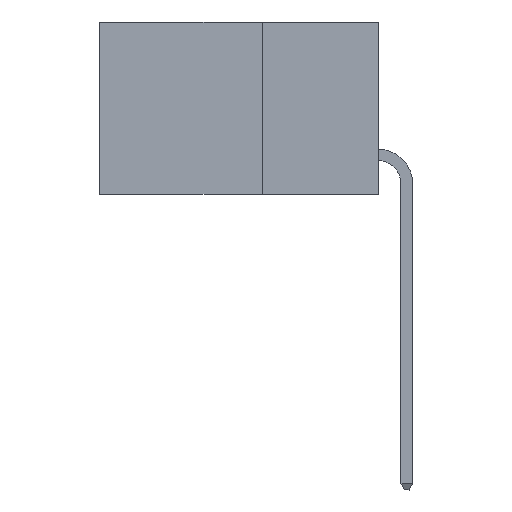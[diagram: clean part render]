
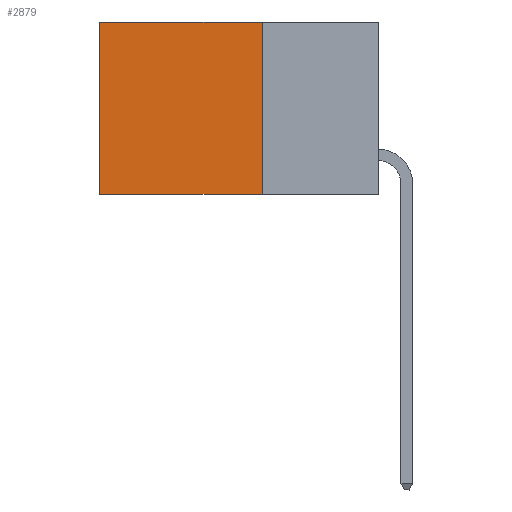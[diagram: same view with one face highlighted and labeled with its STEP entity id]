
A CAD part, left-side view. The second image highlights one B-rep face of the part: STEP entity #2879.
In plain terms, the highlighted planar face has unit normal (-1, 0, 0).
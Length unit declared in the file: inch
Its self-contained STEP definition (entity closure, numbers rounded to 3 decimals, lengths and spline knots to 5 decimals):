
#283 = ORIENTED_EDGE ( 'NONE', *, *, #8008, .T. ) ;
#364 = LINE ( 'NONE', #12319, #1823 ) ;
#633 = FACE_OUTER_BOUND ( 'NONE', #9803, .T. ) ;
#1013 = DIRECTION ( 'NONE',  ( 0., 1., 0. ) ) ;
#1372 = VERTEX_POINT ( 'NONE', #11351 ) ;
#1469 = VERTEX_POINT ( 'NONE', #7396 ) ;
#1823 = VECTOR ( 'NONE', #4928, 39.37008 ) ;
#2589 = DIRECTION ( 'NONE',  ( 0., 0., -1. ) ) ;
#2618 = ORIENTED_EDGE ( 'NONE', *, *, #8713, .F. ) ;
#2879 = ADVANCED_FACE ( 'NONE', ( #633 ), #7696, .F. ) ;
#3606 = VECTOR ( 'NONE', #6591, 39.37008 ) ;
#3637 = LINE ( 'NONE', #9438, #8852 ) ;
#4437 = VERTEX_POINT ( 'NONE', #12358 ) ;
#4906 = LINE ( 'NONE', #5611, #3606 ) ;
#4928 = DIRECTION ( 'NONE',  ( 0., 0., -1. ) ) ;
#5316 = DIRECTION ( 'NONE',  ( 0., 0., -1. ) ) ;
#5583 = DIRECTION ( 'NONE',  ( 1., 0., 0. ) ) ;
#5611 = CARTESIAN_POINT ( 'NONE',  ( 0.298, 0.25, 0. ) ) ;
#6186 = LINE ( 'NONE', #11544, #11407 ) ;
#6591 = DIRECTION ( 'NONE',  ( 0., 1., 0. ) ) ;
#7368 = EDGE_CURVE ( 'NONE', #4437, #1372, #4906, .T. ) ;
#7396 = CARTESIAN_POINT ( 'NONE',  ( 0.298, 0.6, -0.37 ) ) ;
#7447 = CARTESIAN_POINT ( 'NONE',  ( 0.298, 0.25, -0.37 ) ) ;
#7696 = PLANE ( 'NONE',  #12061 ) ;
#8008 = EDGE_CURVE ( 'NONE', #1372, #1469, #6186, .T. ) ;
#8713 = EDGE_CURVE ( 'NONE', #4437, #10358, #364, .T. ) ;
#8852 = VECTOR ( 'NONE', #1013, 39.37008 ) ;
#9438 = CARTESIAN_POINT ( 'NONE',  ( 0.298, 0.25, -0.37 ) ) ;
#9803 = EDGE_LOOP ( 'NONE', ( #283, #12794, #2618, #10281 ) ) ;
#10281 = ORIENTED_EDGE ( 'NONE', *, *, #7368, .T. ) ;
#10358 = VERTEX_POINT ( 'NONE', #7447 ) ;
#11351 = CARTESIAN_POINT ( 'NONE',  ( 0.298, 0.6, 0. ) ) ;
#11407 = VECTOR ( 'NONE', #2589, 39.37008 ) ;
#11544 = CARTESIAN_POINT ( 'NONE',  ( 0.298, 0.6, 0. ) ) ;
#11927 = CARTESIAN_POINT ( 'NONE',  ( 0.298, 0.25, 0. ) ) ;
#12061 = AXIS2_PLACEMENT_3D ( 'NONE', #11927, #5583, #5316 ) ;
#12319 = CARTESIAN_POINT ( 'NONE',  ( 0.298, 0.25, 0. ) ) ;
#12358 = CARTESIAN_POINT ( 'NONE',  ( 0.298, 0.25, 0. ) ) ;
#12794 = ORIENTED_EDGE ( 'NONE', *, *, #12991, .F. ) ;
#12991 = EDGE_CURVE ( 'NONE', #10358, #1469, #3637, .T. ) ;
